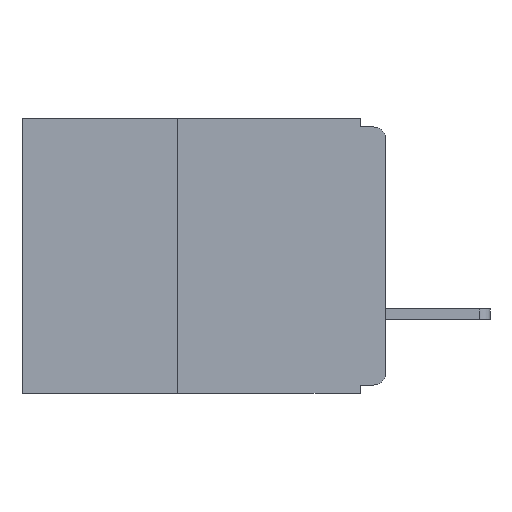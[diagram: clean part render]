
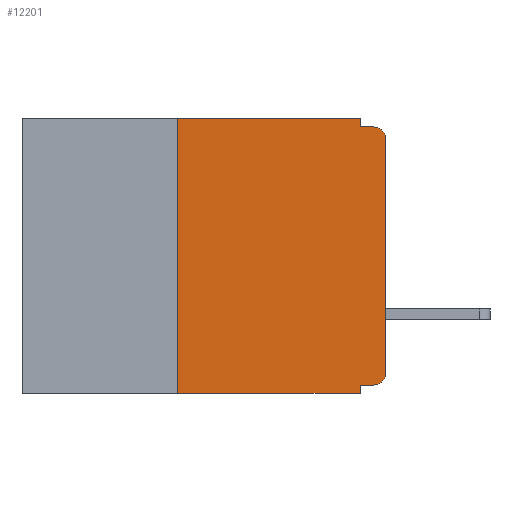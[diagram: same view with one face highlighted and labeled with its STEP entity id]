
A CAD part, left-side view. The second image highlights one B-rep face of the part: STEP entity #12201.
In plain terms, the highlighted planar face has unit normal (-1, 0, 0).
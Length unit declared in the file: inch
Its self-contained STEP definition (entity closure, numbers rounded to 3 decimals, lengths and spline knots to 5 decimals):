
#594 = VERTEX_POINT ( 'NONE', #18589 ) ;
#812 = CARTESIAN_POINT ( 'NONE',  ( 0., 0.25, -0.33 ) ) ;
#951 = VERTEX_POINT ( 'NONE', #9219 ) ;
#1320 = VERTEX_POINT ( 'NONE', #18203 ) ;
#1416 = VECTOR ( 'NONE', #14369, 39.37008 ) ;
#1459 = EDGE_CURVE ( 'NONE', #1320, #2867, #2930, .T. ) ;
#1820 = LINE ( 'NONE', #14434, #1416 ) ;
#1935 = VERTEX_POINT ( 'NONE', #17645 ) ;
#2517 = AXIS2_PLACEMENT_3D ( 'NONE', #4451, #3621, #3543 ) ;
#2608 = ORIENTED_EDGE ( 'NONE', *, *, #17558, .F. ) ;
#2755 = FACE_OUTER_BOUND ( 'NONE', #14449, .T. ) ;
#2818 = VECTOR ( 'NONE', #9129, 39.37008 ) ;
#2867 = VERTEX_POINT ( 'NONE', #19348 ) ;
#2930 = LINE ( 'NONE', #8578, #2818 ) ;
#3181 = CARTESIAN_POINT ( 'NONE',  ( 0., 0., -0.305 ) ) ;
#3205 = DIRECTION ( 'NONE',  ( 0., 0., -1. ) ) ;
#3311 = VECTOR ( 'NONE', #6744, 39.37008 ) ;
#3391 = LINE ( 'NONE', #6776, #3311 ) ;
#3413 = DIRECTION ( 'NONE',  ( -1., 0., 0. ) ) ;
#3543 = DIRECTION ( 'NONE',  ( 0., 0., -1. ) ) ;
#3621 = DIRECTION ( 'NONE',  ( 1., 0., 0. ) ) ;
#3675 = CARTESIAN_POINT ( 'NONE',  ( 0., 0.015, -0.305 ) ) ;
#3684 = VECTOR ( 'NONE', #12421, 39.37008 ) ;
#3784 = PLANE ( 'NONE',  #2517 ) ;
#4004 = LINE ( 'NONE', #12354, #3684 ) ;
#4451 = CARTESIAN_POINT ( 'NONE',  ( 0., 0.437, 0. ) ) ;
#4754 = ORIENTED_EDGE ( 'NONE', *, *, #10538, .T. ) ;
#5489 = VERTEX_POINT ( 'NONE', #3181 ) ;
#5915 = EDGE_CURVE ( 'NONE', #951, #1935, #4004, .T. ) ;
#5925 = CARTESIAN_POINT ( 'NONE',  ( 0., 0.015, -0.32 ) ) ;
#6222 = AXIS2_PLACEMENT_3D ( 'NONE', #3675, #3413, #3205 ) ;
#6744 = DIRECTION ( 'NONE',  ( 0., 0., -1. ) ) ;
#6766 = VERTEX_POINT ( 'NONE', #10354 ) ;
#6776 = CARTESIAN_POINT ( 'NONE',  ( 0., 0.031, 0. ) ) ;
#6899 = CARTESIAN_POINT ( 'NONE',  ( 0., 0.031, -0.32 ) ) ;
#6924 = EDGE_CURVE ( 'NONE', #6766, #2867, #7129, .T. ) ;
#7020 = LINE ( 'NONE', #13889, #7159 ) ;
#7129 = CIRCLE ( 'NONE', #16010, 0.015 ) ;
#7159 = VECTOR ( 'NONE', #13991, 39.37008 ) ;
#7247 = ORIENTED_EDGE ( 'NONE', *, *, #8221, .T. ) ;
#7434 = ORIENTED_EDGE ( 'NONE', *, *, #18594, .T. ) ;
#7448 = ORIENTED_EDGE ( 'NONE', *, *, #17914, .F. ) ;
#8221 = EDGE_CURVE ( 'NONE', #8982, #594, #1820, .T. ) ;
#8578 = CARTESIAN_POINT ( 'NONE',  ( 0., 0., -0.01 ) ) ;
#8720 = ORIENTED_EDGE ( 'NONE', *, *, #6924, .T. ) ;
#8982 = VERTEX_POINT ( 'NONE', #812 ) ;
#9129 = DIRECTION ( 'NONE',  ( 0., -1., 0. ) ) ;
#9219 = CARTESIAN_POINT ( 'NONE',  ( 0., 0.25, 0. ) ) ;
#9619 = VERTEX_POINT ( 'NONE', #5925 ) ;
#10354 = CARTESIAN_POINT ( 'NONE',  ( 0., 0., -0.025 ) ) ;
#10538 = EDGE_CURVE ( 'NONE', #9619, #5489, #11307, .T. ) ;
#10684 = ORIENTED_EDGE ( 'NONE', *, *, #1459, .F. ) ;
#10806 = VECTOR ( 'NONE', #12549, 39.37008 ) ;
#10830 = LINE ( 'NONE', #12571, #10806 ) ;
#11307 = CIRCLE ( 'NONE', #6222, 0.015 ) ;
#11389 = ORIENTED_EDGE ( 'NONE', *, *, #16333, .F. ) ;
#11635 = ORIENTED_EDGE ( 'NONE', *, *, #5915, .F. ) ;
#12201 = ADVANCED_FACE ( 'NONE', ( #2755 ), #3784, .F. ) ;
#12354 = CARTESIAN_POINT ( 'NONE',  ( 0., 0.437, 0. ) ) ;
#12421 = DIRECTION ( 'NONE',  ( 0., -1., 0. ) ) ;
#12549 = DIRECTION ( 'NONE',  ( 0., 0., 1. ) ) ;
#12571 = CARTESIAN_POINT ( 'NONE',  ( 0., 0., 0. ) ) ;
#13328 = DIRECTION ( 'NONE',  ( 0., 0., -1. ) ) ;
#13685 = CARTESIAN_POINT ( 'NONE',  ( 0., 0.031, -0.33 ) ) ;
#13889 = CARTESIAN_POINT ( 'NONE',  ( 0., 0.25, -0.33 ) ) ;
#13991 = DIRECTION ( 'NONE',  ( 0., 0., 1. ) ) ;
#14369 = DIRECTION ( 'NONE',  ( 0., -1., 0. ) ) ;
#14424 = EDGE_CURVE ( 'NONE', #8982, #951, #7020, .T. ) ;
#14434 = CARTESIAN_POINT ( 'NONE',  ( 0., 0.437, -0.33 ) ) ;
#14449 = EDGE_LOOP ( 'NONE', ( #7434, #8720, #10684, #11389, #11635, #15570, #7247, #2608, #7448, #4754 ) ) ;
#14489 = VECTOR ( 'NONE', #15723, 39.37008 ) ;
#14587 = LINE ( 'NONE', #15741, #14489 ) ;
#15570 = ORIENTED_EDGE ( 'NONE', *, *, #14424, .F. ) ;
#15723 = DIRECTION ( 'NONE',  ( 0., 1., 0. ) ) ;
#15741 = CARTESIAN_POINT ( 'NONE',  ( 0., 0., -0.32 ) ) ;
#16010 = AXIS2_PLACEMENT_3D ( 'NONE', #18332, #18328, #18316 ) ;
#16333 = EDGE_CURVE ( 'NONE', #1935, #1320, #3391, .T. ) ;
#16641 = VECTOR ( 'NONE', #13328, 39.37008 ) ;
#16742 = LINE ( 'NONE', #13685, #16641 ) ;
#17558 = EDGE_CURVE ( 'NONE', #19495, #594, #16742, .T. ) ;
#17645 = CARTESIAN_POINT ( 'NONE',  ( 0., 0.031, 0. ) ) ;
#17914 = EDGE_CURVE ( 'NONE', #9619, #19495, #14587, .T. ) ;
#18203 = CARTESIAN_POINT ( 'NONE',  ( 0., 0.031, -0.01 ) ) ;
#18316 = DIRECTION ( 'NONE',  ( 0., 0., -1. ) ) ;
#18328 = DIRECTION ( 'NONE',  ( -1., 0., 0. ) ) ;
#18332 = CARTESIAN_POINT ( 'NONE',  ( 0., 0.015, -0.025 ) ) ;
#18589 = CARTESIAN_POINT ( 'NONE',  ( 0., 0.031, -0.33 ) ) ;
#18594 = EDGE_CURVE ( 'NONE', #5489, #6766, #10830, .T. ) ;
#19348 = CARTESIAN_POINT ( 'NONE',  ( 0., 0.015, -0.01 ) ) ;
#19495 = VERTEX_POINT ( 'NONE', #6899 ) ;
